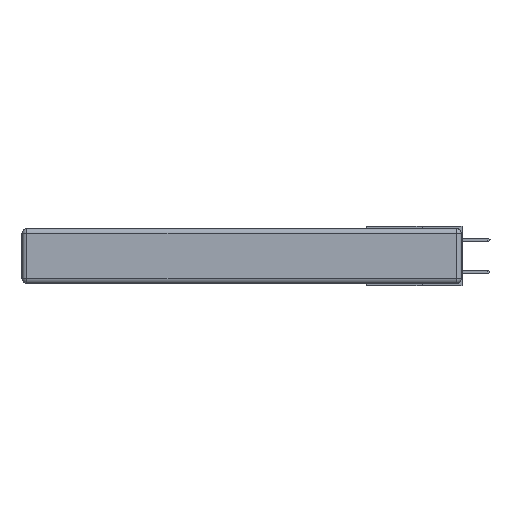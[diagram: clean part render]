
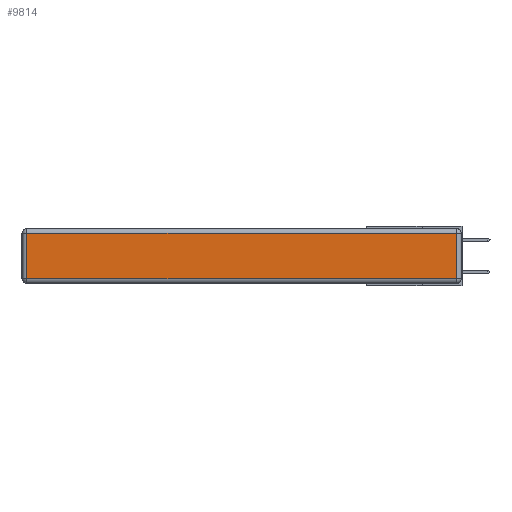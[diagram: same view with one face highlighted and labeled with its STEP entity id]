
A CAD part, left-side view. The second image highlights one B-rep face of the part: STEP entity #9814.
In plain terms, the highlighted planar face has unit normal (-1, 0, 0).
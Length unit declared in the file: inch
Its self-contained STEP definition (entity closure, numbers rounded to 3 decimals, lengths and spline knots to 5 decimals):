
#974 = ORIENTED_EDGE ( 'NONE', *, *, #6898, .T. ) ;
#1187 = CARTESIAN_POINT ( 'NONE',  ( 0., 0.03, -0.343 ) ) ;
#1370 = VECTOR ( 'NONE', #14388, 39.37008 ) ;
#1680 = DIRECTION ( 'NONE',  ( 0., -1., 0. ) ) ;
#2374 = CARTESIAN_POINT ( 'NONE',  ( 0., 2.72, -0.313 ) ) ;
#2410 = CARTESIAN_POINT ( 'NONE',  ( 0., 2.75, -0.03 ) ) ;
#3107 = LINE ( 'NONE', #4547, #10990 ) ;
#4547 = CARTESIAN_POINT ( 'NONE',  ( 0., 2.72, -0.343 ) ) ;
#5207 = VECTOR ( 'NONE', #1680, 39.37008 ) ;
#5364 = AXIS2_PLACEMENT_3D ( 'NONE', #7989, #12486, #7754 ) ;
#6021 = VERTEX_POINT ( 'NONE', #15599 ) ;
#6162 = EDGE_CURVE ( 'NONE', #10651, #19034, #16893, .T. ) ;
#6898 = EDGE_CURVE ( 'NONE', #6021, #10651, #13177, .T. ) ;
#7536 = DIRECTION ( 'NONE',  ( 0., 0., -1. ) ) ;
#7754 = DIRECTION ( 'NONE',  ( 0., 0., 1. ) ) ;
#7989 = CARTESIAN_POINT ( 'NONE',  ( 0., 0., -0.343 ) ) ;
#8809 = EDGE_CURVE ( 'NONE', #19034, #16522, #3107, .T. ) ;
#9199 = VECTOR ( 'NONE', #13138, 39.37008 ) ;
#9814 = ADVANCED_FACE ( 'NONE', ( #17481 ), #18206, .T. ) ;
#10651 = VERTEX_POINT ( 'NONE', #18441 ) ;
#10990 = VECTOR ( 'NONE', #7536, 39.37008 ) ;
#12265 = ORIENTED_EDGE ( 'NONE', *, *, #6162, .T. ) ;
#12486 = DIRECTION ( 'NONE',  ( -1., 0., 0. ) ) ;
#13138 = DIRECTION ( 'NONE',  ( 0., 0., 1. ) ) ;
#13177 = LINE ( 'NONE', #1187, #9199 ) ;
#14026 = CARTESIAN_POINT ( 'NONE',  ( 0., 2.72, -0.03 ) ) ;
#14388 = DIRECTION ( 'NONE',  ( 0., 1., 0. ) ) ;
#15132 = ORIENTED_EDGE ( 'NONE', *, *, #15369, .T. ) ;
#15369 = EDGE_CURVE ( 'NONE', #16522, #6021, #18483, .T. ) ;
#15487 = ORIENTED_EDGE ( 'NONE', *, *, #8809, .T. ) ;
#15599 = CARTESIAN_POINT ( 'NONE',  ( 0., 0.03, -0.313 ) ) ;
#16522 = VERTEX_POINT ( 'NONE', #2374 ) ;
#16893 = LINE ( 'NONE', #2410, #1370 ) ;
#17481 = FACE_OUTER_BOUND ( 'NONE', #17853, .T. ) ;
#17853 = EDGE_LOOP ( 'NONE', ( #15132, #974, #12265, #15487 ) ) ;
#18109 = CARTESIAN_POINT ( 'NONE',  ( 0., 0., -0.313 ) ) ;
#18206 = PLANE ( 'NONE',  #5364 ) ;
#18441 = CARTESIAN_POINT ( 'NONE',  ( 0., 0.03, -0.03 ) ) ;
#18483 = LINE ( 'NONE', #18109, #5207 ) ;
#19034 = VERTEX_POINT ( 'NONE', #14026 ) ;
